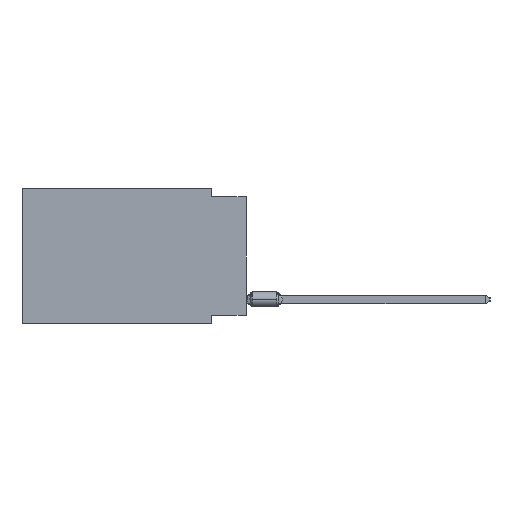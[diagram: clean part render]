
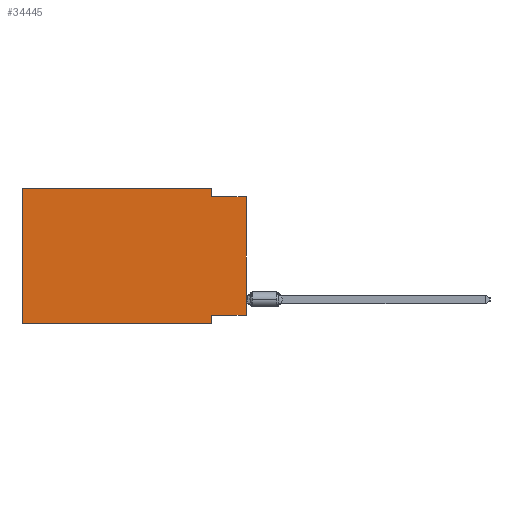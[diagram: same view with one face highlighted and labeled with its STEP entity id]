
A CAD part, left-side view. The second image highlights one B-rep face of the part: STEP entity #34445.
In plain terms, the highlighted planar face has unit normal (-1, 0, 0).
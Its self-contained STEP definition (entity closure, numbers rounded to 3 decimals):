
#143 = LINE ( 'NONE', #33306, #36333 ) ;
#866 = EDGE_CURVE ( 'NONE', #38650, #16019, #36761, .T. ) ;
#1025 = VERTEX_POINT ( 'NONE', #37925 ) ;
#1096 = VECTOR ( 'NONE', #9682, 1000. ) ;
#1486 = EDGE_CURVE ( 'NONE', #38650, #1025, #4571, .T. ) ;
#1702 = PLANE ( 'NONE',  #21902 ) ;
#3239 = CARTESIAN_POINT ( 'NONE',  ( 0., 2.54, 0. ) ) ;
#4571 = LINE ( 'NONE', #13974, #28104 ) ;
#4657 = DIRECTION ( 'NONE',  ( 0., 0., -1. ) ) ;
#5266 = LINE ( 'NONE', #29420, #24128 ) ;
#5563 = LINE ( 'NONE', #14168, #19459 ) ;
#6021 = DIRECTION ( 'NONE',  ( 0., 0., 1. ) ) ;
#6381 = LINE ( 'NONE', #18329, #6982 ) ;
#6982 = VECTOR ( 'NONE', #21836, 1000. ) ;
#7532 = EDGE_CURVE ( 'NONE', #14315, #19991, #38123, .T. ) ;
#8071 = ORIENTED_EDGE ( 'NONE', *, *, #17483, .F. ) ;
#8351 = ORIENTED_EDGE ( 'NONE', *, *, #35400, .F. ) ;
#9682 = DIRECTION ( 'NONE',  ( 0., 0., 1. ) ) ;
#10158 = CARTESIAN_POINT ( 'NONE',  ( 0., 16.383, 0. ) ) ;
#12595 = EDGE_CURVE ( 'NONE', #22605, #30668, #143, .T. ) ;
#12839 = CARTESIAN_POINT ( 'NONE',  ( 0., 0., -9.271 ) ) ;
#13569 = DIRECTION ( 'NONE',  ( 0., -1., 0. ) ) ;
#13974 = CARTESIAN_POINT ( 'NONE',  ( 0., 16.383, -9.906 ) ) ;
#14168 = CARTESIAN_POINT ( 'NONE',  ( 0., 0., -0.635 ) ) ;
#14195 = ORIENTED_EDGE ( 'NONE', *, *, #19495, .F. ) ;
#14315 = VERTEX_POINT ( 'NONE', #3239 ) ;
#15835 = ORIENTED_EDGE ( 'NONE', *, *, #12595, .T. ) ;
#16019 = VERTEX_POINT ( 'NONE', #25914 ) ;
#17483 = EDGE_CURVE ( 'NONE', #31363, #1025, #18650, .T. ) ;
#17713 = DIRECTION ( 'NONE',  ( 0., 0., -1. ) ) ;
#18003 = EDGE_LOOP ( 'NONE', ( #15835, #8351, #35511, #14195, #28253, #31036, #8071, #37091 ) ) ;
#18329 = CARTESIAN_POINT ( 'NONE',  ( 0., 0., -9.271 ) ) ;
#18650 = LINE ( 'NONE', #33785, #37993 ) ;
#18858 = DIRECTION ( 'NONE',  ( 0., 0., -1. ) ) ;
#19459 = VECTOR ( 'NONE', #23001, 1000. ) ;
#19495 = EDGE_CURVE ( 'NONE', #16019, #14315, #5266, .T. ) ;
#19748 = DIRECTION ( 'NONE',  ( 0., -1., 0. ) ) ;
#19991 = VERTEX_POINT ( 'NONE', #38183 ) ;
#21836 = DIRECTION ( 'NONE',  ( 0., 1., 0. ) ) ;
#21902 = AXIS2_PLACEMENT_3D ( 'NONE', #10158, #34289, #4657 ) ;
#22605 = VERTEX_POINT ( 'NONE', #12839 ) ;
#23001 = DIRECTION ( 'NONE',  ( 0., -1., 0. ) ) ;
#24128 = VECTOR ( 'NONE', #19748, 1000. ) ;
#25432 = FACE_OUTER_BOUND ( 'NONE', #18003, .T. ) ;
#25914 = CARTESIAN_POINT ( 'NONE',  ( 0., 16.383, 0. ) ) ;
#26249 = VECTOR ( 'NONE', #17713, 1000. ) ;
#27778 = CARTESIAN_POINT ( 'NONE',  ( 0., 0., -0.635 ) ) ;
#28104 = VECTOR ( 'NONE', #13569, 1000. ) ;
#28253 = ORIENTED_EDGE ( 'NONE', *, *, #866, .F. ) ;
#29420 = CARTESIAN_POINT ( 'NONE',  ( 0., 16.383, 0. ) ) ;
#30668 = VERTEX_POINT ( 'NONE', #27778 ) ;
#31036 = ORIENTED_EDGE ( 'NONE', *, *, #1486, .T. ) ;
#31272 = CARTESIAN_POINT ( 'NONE',  ( 0., 16.383, 0. ) ) ;
#31363 = VERTEX_POINT ( 'NONE', #37077 ) ;
#32651 = CARTESIAN_POINT ( 'NONE',  ( 0., 2.54, 0. ) ) ;
#33284 = CARTESIAN_POINT ( 'NONE',  ( 0., 16.383, -9.906 ) ) ;
#33306 = CARTESIAN_POINT ( 'NONE',  ( 0., 0., 0. ) ) ;
#33785 = CARTESIAN_POINT ( 'NONE',  ( 0., 2.54, -9.906 ) ) ;
#34289 = DIRECTION ( 'NONE',  ( 1., 0., 0. ) ) ;
#34445 = ADVANCED_FACE ( 'NONE', ( #25432 ), #1702, .F. ) ;
#35400 = EDGE_CURVE ( 'NONE', #19991, #30668, #5563, .T. ) ;
#35511 = ORIENTED_EDGE ( 'NONE', *, *, #7532, .F. ) ;
#35904 = EDGE_CURVE ( 'NONE', #22605, #31363, #6381, .T. ) ;
#36333 = VECTOR ( 'NONE', #6021, 1000. ) ;
#36761 = LINE ( 'NONE', #31272, #1096 ) ;
#37077 = CARTESIAN_POINT ( 'NONE',  ( 0., 2.54, -9.271 ) ) ;
#37091 = ORIENTED_EDGE ( 'NONE', *, *, #35904, .F. ) ;
#37925 = CARTESIAN_POINT ( 'NONE',  ( 0., 2.54, -9.906 ) ) ;
#37993 = VECTOR ( 'NONE', #18858, 1000. ) ;
#38123 = LINE ( 'NONE', #32651, #26249 ) ;
#38183 = CARTESIAN_POINT ( 'NONE',  ( 0., 2.54, -0.635 ) ) ;
#38650 = VERTEX_POINT ( 'NONE', #33284 ) ;
